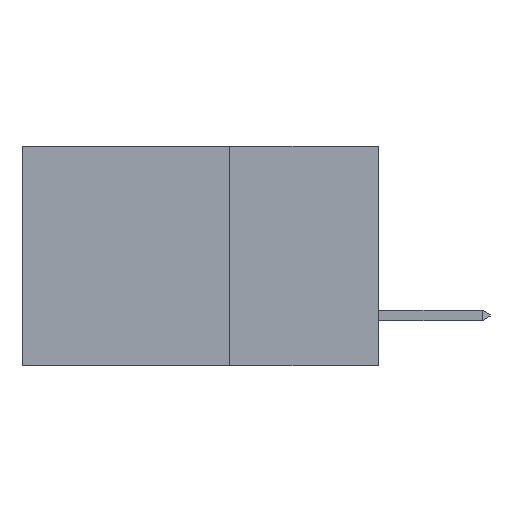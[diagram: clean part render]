
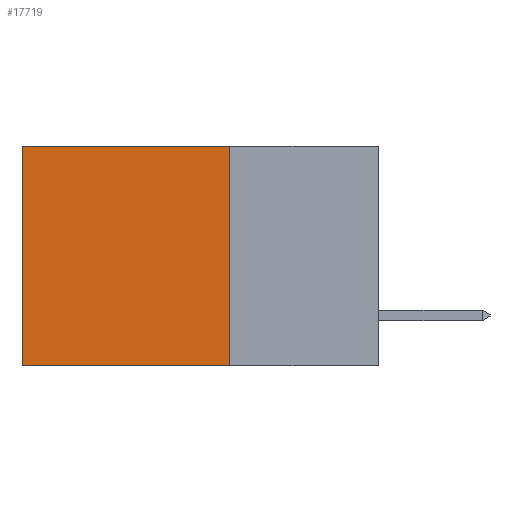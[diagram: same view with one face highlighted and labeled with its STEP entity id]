
A CAD part, left-side view. The second image highlights one B-rep face of the part: STEP entity #17719.
In plain terms, the highlighted planar face has unit normal (-1, 0, 0).
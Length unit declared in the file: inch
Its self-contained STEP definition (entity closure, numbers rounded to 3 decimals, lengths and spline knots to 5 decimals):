
#1732 = LINE ( 'NONE', #14870, #12562 ) ;
#2210 = VECTOR ( 'NONE', #23455, 39.37008 ) ;
#2369 = CARTESIAN_POINT ( 'NONE',  ( 0.298, 0.6, 0. ) ) ;
#2663 = EDGE_CURVE ( 'NONE', #10260, #13612, #21998, .T. ) ;
#4192 = CARTESIAN_POINT ( 'NONE',  ( 0.298, 0.25, 0. ) ) ;
#4972 = VECTOR ( 'NONE', #18495, 39.37008 ) ;
#5433 = EDGE_CURVE ( 'NONE', #10260, #19375, #1732, .T. ) ;
#5614 = CARTESIAN_POINT ( 'NONE',  ( 0.298, 0.6, -0.37 ) ) ;
#6208 = ORIENTED_EDGE ( 'NONE', *, *, #5433, .T. ) ;
#6740 = CARTESIAN_POINT ( 'NONE',  ( 0.298, 0.25, 0. ) ) ;
#7552 = FACE_OUTER_BOUND ( 'NONE', #16231, .T. ) ;
#8587 = CARTESIAN_POINT ( 'NONE',  ( 0.298, 0.25, -0.37 ) ) ;
#10260 = VERTEX_POINT ( 'NONE', #4192 ) ;
#11024 = DIRECTION ( 'NONE',  ( 0., 0., -1. ) ) ;
#11730 = AXIS2_PLACEMENT_3D ( 'NONE', #6740, #23715, #11024 ) ;
#11785 = LINE ( 'NONE', #2369, #17467 ) ;
#12319 = ORIENTED_EDGE ( 'NONE', *, *, #20463, .T. ) ;
#12562 = VECTOR ( 'NONE', #14364, 39.37008 ) ;
#12975 = ORIENTED_EDGE ( 'NONE', *, *, #2663, .F. ) ;
#13066 = DIRECTION ( 'NONE',  ( 0., 0., -1. ) ) ;
#13612 = VERTEX_POINT ( 'NONE', #26427 ) ;
#14068 = CARTESIAN_POINT ( 'NONE',  ( 0.298, 0.6, 0. ) ) ;
#14364 = DIRECTION ( 'NONE',  ( 0., 1., 0. ) ) ;
#14870 = CARTESIAN_POINT ( 'NONE',  ( 0.298, 0.25, 0. ) ) ;
#15826 = EDGE_CURVE ( 'NONE', #13612, #17520, #19362, .T. ) ;
#16231 = EDGE_LOOP ( 'NONE', ( #12319, #17795, #12975, #6208 ) ) ;
#17224 = CARTESIAN_POINT ( 'NONE',  ( 0.298, 0.25, 0. ) ) ;
#17467 = VECTOR ( 'NONE', #13066, 39.37008 ) ;
#17520 = VERTEX_POINT ( 'NONE', #5614 ) ;
#17719 = ADVANCED_FACE ( 'NONE', ( #7552 ), #19518, .F. ) ;
#17795 = ORIENTED_EDGE ( 'NONE', *, *, #15826, .F. ) ;
#18495 = DIRECTION ( 'NONE',  ( 0., 0., -1. ) ) ;
#19362 = LINE ( 'NONE', #8587, #2210 ) ;
#19375 = VERTEX_POINT ( 'NONE', #14068 ) ;
#19518 = PLANE ( 'NONE',  #11730 ) ;
#20463 = EDGE_CURVE ( 'NONE', #19375, #17520, #11785, .T. ) ;
#21998 = LINE ( 'NONE', #17224, #4972 ) ;
#23455 = DIRECTION ( 'NONE',  ( 0., 1., 0. ) ) ;
#23715 = DIRECTION ( 'NONE',  ( 1., 0., 0. ) ) ;
#26427 = CARTESIAN_POINT ( 'NONE',  ( 0.298, 0.25, -0.37 ) ) ;
